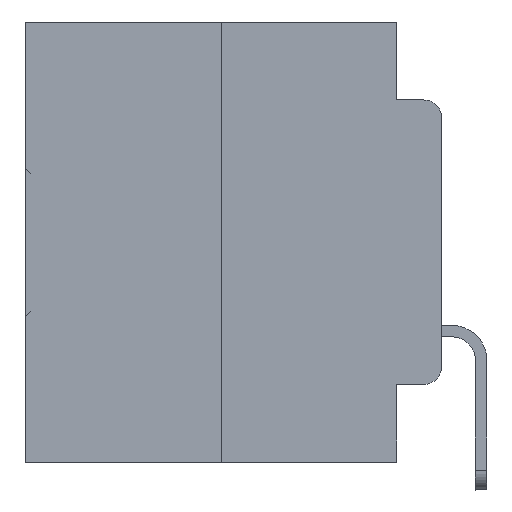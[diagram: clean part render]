
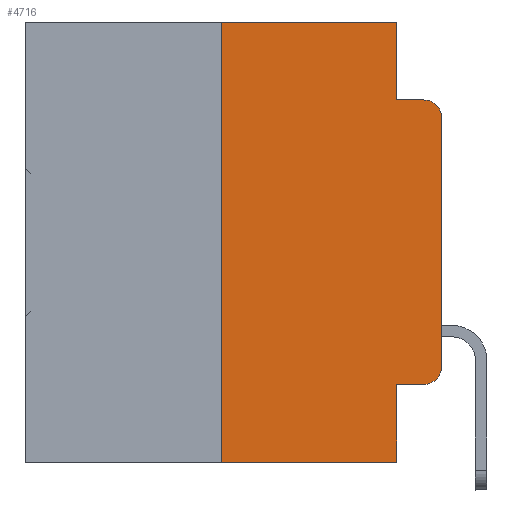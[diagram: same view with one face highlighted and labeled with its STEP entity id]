
A CAD part, left-side view. The second image highlights one B-rep face of the part: STEP entity #4716.
In plain terms, the highlighted planar face has unit normal (-1, 0, 0).
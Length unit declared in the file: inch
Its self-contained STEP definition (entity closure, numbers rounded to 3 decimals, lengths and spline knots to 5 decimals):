
#896 = DIRECTION ( 'NONE',  ( 0., -1., 0. ) ) ;
#1693 = CARTESIAN_POINT ( 'NONE',  ( 0., 0.473, 0. ) ) ;
#1877 = LINE ( 'NONE', #14797, #8365 ) ;
#2330 = EDGE_CURVE ( 'NONE', #16768, #18979, #12696, .T. ) ;
#2547 = VERTEX_POINT ( 'NONE', #24094 ) ;
#2921 = VECTOR ( 'NONE', #10925, 39.37008 ) ;
#3068 = EDGE_CURVE ( 'NONE', #2547, #25923, #27831, .T. ) ;
#3179 = VERTEX_POINT ( 'NONE', #4411 ) ;
#3246 = CARTESIAN_POINT ( 'NONE',  ( 0., 0.25, 0. ) ) ;
#3313 = DIRECTION ( 'NONE',  ( 0., 0., -1. ) ) ;
#3707 = AXIS2_PLACEMENT_3D ( 'NONE', #24052, #21549, #18865 ) ;
#4411 = CARTESIAN_POINT ( 'NONE',  ( 0., 0.25, -0.5 ) ) ;
#4716 = ADVANCED_FACE ( 'NONE', ( #8590 ), #24685, .F. ) ;
#4886 = ORIENTED_EDGE ( 'NONE', *, *, #24956, .T. ) ;
#4985 = CARTESIAN_POINT ( 'NONE',  ( 0., 0.051, -0.4115 ) ) ;
#6449 = CARTESIAN_POINT ( 'NONE',  ( 0., 0.473, -0.5 ) ) ;
#6768 = LINE ( 'NONE', #6449, #12056 ) ;
#8365 = VECTOR ( 'NONE', #9438, 39.37008 ) ;
#8590 = FACE_OUTER_BOUND ( 'NONE', #29840, .T. ) ;
#8810 = CARTESIAN_POINT ( 'NONE',  ( 0., 0.473, 0. ) ) ;
#9438 = DIRECTION ( 'NONE',  ( 0., 0., 1. ) ) ;
#9800 = LINE ( 'NONE', #20047, #27967 ) ;
#10130 = LINE ( 'NONE', #20375, #11619 ) ;
#10863 = CARTESIAN_POINT ( 'NONE',  ( 0., 0.02, -0.3915 ) ) ;
#10925 = DIRECTION ( 'NONE',  ( 0., 0., -1. ) ) ;
#11600 = DIRECTION ( 'NONE',  ( 1., 0., 0. ) ) ;
#11619 = VECTOR ( 'NONE', #30617, 39.37008 ) ;
#11959 = ORIENTED_EDGE ( 'NONE', *, *, #26763, .F. ) ;
#12056 = VECTOR ( 'NONE', #896, 39.37008 ) ;
#12415 = CIRCLE ( 'NONE', #18847, 0.02 ) ;
#12696 = LINE ( 'NONE', #4985, #32686 ) ;
#13400 = ORIENTED_EDGE ( 'NONE', *, *, #23330, .F. ) ;
#13476 = VERTEX_POINT ( 'NONE', #33000 ) ;
#13695 = CARTESIAN_POINT ( 'NONE',  ( 0., 0., -0.3915 ) ) ;
#13783 = LINE ( 'NONE', #31247, #2921 ) ;
#13814 = VECTOR ( 'NONE', #29994, 39.37008 ) ;
#14224 = EDGE_CURVE ( 'NONE', #31245, #25923, #17072, .T. ) ;
#14512 = ORIENTED_EDGE ( 'NONE', *, *, #2330, .T. ) ;
#14700 = CARTESIAN_POINT ( 'NONE',  ( 0., 0.02, -0.0885 ) ) ;
#14797 = CARTESIAN_POINT ( 'NONE',  ( 0., 0.25, 0. ) ) ;
#16768 = VERTEX_POINT ( 'NONE', #29557 ) ;
#16841 = ORIENTED_EDGE ( 'NONE', *, *, #26058, .F. ) ;
#16856 = CARTESIAN_POINT ( 'NONE',  ( 0., 0.051, -0.0885 ) ) ;
#17072 = LINE ( 'NONE', #20094, #13814 ) ;
#17449 = VERTEX_POINT ( 'NONE', #3246 ) ;
#18847 = AXIS2_PLACEMENT_3D ( 'NONE', #10863, #26299, #3313 ) ;
#18865 = DIRECTION ( 'NONE',  ( 0., 0., -1. ) ) ;
#18979 = VERTEX_POINT ( 'NONE', #21060 ) ;
#19806 = EDGE_CURVE ( 'NONE', #18979, #29634, #12415, .T. ) ;
#20047 = CARTESIAN_POINT ( 'NONE',  ( 0., 0., 0. ) ) ;
#20094 = CARTESIAN_POINT ( 'NONE',  ( 0., 0.051, -0.0885 ) ) ;
#20375 = CARTESIAN_POINT ( 'NONE',  ( 0., 0.051, 0. ) ) ;
#20435 = EDGE_CURVE ( 'NONE', #29634, #2547, #9800, .T. ) ;
#20469 = ORIENTED_EDGE ( 'NONE', *, *, #20435, .T. ) ;
#21060 = CARTESIAN_POINT ( 'NONE',  ( 0., 0.02, -0.4115 ) ) ;
#21340 = DIRECTION ( 'NONE',  ( 0., 0., -1. ) ) ;
#21549 = DIRECTION ( 'NONE',  ( -1., 0., 0. ) ) ;
#21579 = ORIENTED_EDGE ( 'NONE', *, *, #3068, .T. ) ;
#21902 = LINE ( 'NONE', #8810, #22851 ) ;
#22851 = VECTOR ( 'NONE', #26764, 39.37008 ) ;
#23330 = EDGE_CURVE ( 'NONE', #16768, #24432, #13783, .T. ) ;
#24052 = CARTESIAN_POINT ( 'NONE',  ( 0., 0.02, -0.1085 ) ) ;
#24094 = CARTESIAN_POINT ( 'NONE',  ( 0., 0., -0.1085 ) ) ;
#24269 = CARTESIAN_POINT ( 'NONE',  ( 0., 0.051, -0.5 ) ) ;
#24432 = VERTEX_POINT ( 'NONE', #24269 ) ;
#24685 = PLANE ( 'NONE',  #28455 ) ;
#24956 = EDGE_CURVE ( 'NONE', #3179, #24432, #6768, .T. ) ;
#25763 = ORIENTED_EDGE ( 'NONE', *, *, #19806, .T. ) ;
#25923 = VERTEX_POINT ( 'NONE', #14700 ) ;
#26058 = EDGE_CURVE ( 'NONE', #3179, #17449, #1877, .T. ) ;
#26299 = DIRECTION ( 'NONE',  ( -1., 0., 0. ) ) ;
#26544 = EDGE_CURVE ( 'NONE', #17449, #13476, #21902, .T. ) ;
#26763 = EDGE_CURVE ( 'NONE', #13476, #31245, #10130, .T. ) ;
#26764 = DIRECTION ( 'NONE',  ( 0., -1., 0. ) ) ;
#27831 = CIRCLE ( 'NONE', #3707, 0.02 ) ;
#27967 = VECTOR ( 'NONE', #30282, 39.37008 ) ;
#28308 = DIRECTION ( 'NONE',  ( 0., -1., 0. ) ) ;
#28455 = AXIS2_PLACEMENT_3D ( 'NONE', #1693, #11600, #21340 ) ;
#29260 = ORIENTED_EDGE ( 'NONE', *, *, #14224, .F. ) ;
#29557 = CARTESIAN_POINT ( 'NONE',  ( 0., 0.051, -0.4115 ) ) ;
#29634 = VERTEX_POINT ( 'NONE', #13695 ) ;
#29840 = EDGE_LOOP ( 'NONE', ( #20469, #21579, #29260, #11959, #31665, #16841, #4886, #13400, #14512, #25763 ) ) ;
#29994 = DIRECTION ( 'NONE',  ( 0., -1., 0. ) ) ;
#30282 = DIRECTION ( 'NONE',  ( 0., 0., 1. ) ) ;
#30617 = DIRECTION ( 'NONE',  ( 0., 0., -1. ) ) ;
#31245 = VERTEX_POINT ( 'NONE', #16856 ) ;
#31247 = CARTESIAN_POINT ( 'NONE',  ( 0., 0.051, 0. ) ) ;
#31665 = ORIENTED_EDGE ( 'NONE', *, *, #26544, .F. ) ;
#32686 = VECTOR ( 'NONE', #28308, 39.37008 ) ;
#33000 = CARTESIAN_POINT ( 'NONE',  ( 0., 0.051, 0. ) ) ;
